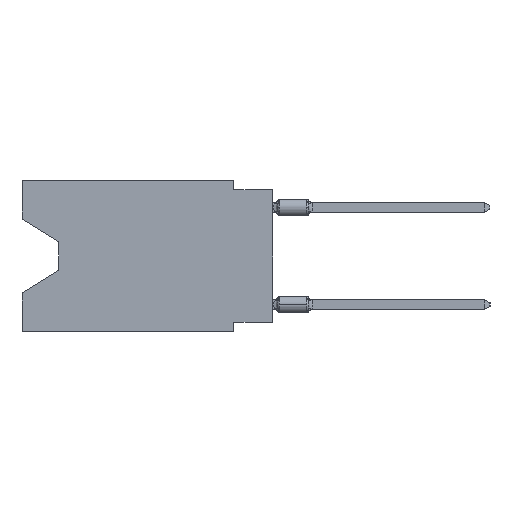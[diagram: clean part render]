
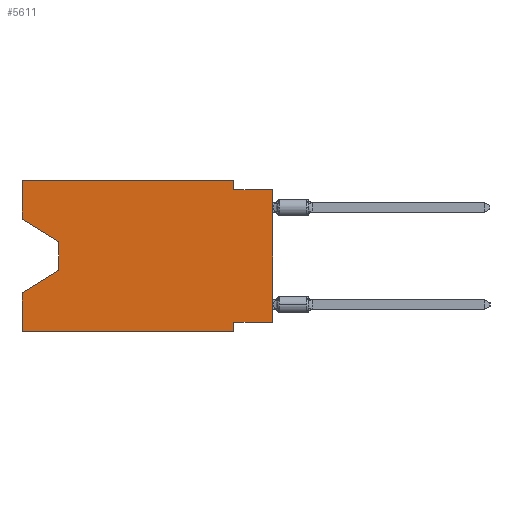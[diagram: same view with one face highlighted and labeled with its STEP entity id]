
A CAD part, left-side view. The second image highlights one B-rep face of the part: STEP entity #5611.
In plain terms, the highlighted planar face has unit normal (-1, 0, 0).
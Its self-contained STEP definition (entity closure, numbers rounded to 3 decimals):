
#142 = ORIENTED_EDGE ( 'NONE', *, *, #10924, .F. ) ;
#152 = VERTEX_POINT ( 'NONE', #18323 ) ;
#203 = VERTEX_POINT ( 'NONE', #12142 ) ;
#2177 = ORIENTED_EDGE ( 'NONE', *, *, #13288, .F. ) ;
#2533 = LINE ( 'NONE', #10088, #13872 ) ;
#2876 = DIRECTION ( 'NONE',  ( 0., 0., 1. ) ) ;
#3063 = PLANE ( 'NONE',  #28915 ) ;
#3248 = DIRECTION ( 'NONE',  ( 0., -1., 0. ) ) ;
#3420 = LINE ( 'NONE', #3580, #19638 ) ;
#3467 = CARTESIAN_POINT ( 'NONE',  ( 0., 16.383, 0. ) ) ;
#3580 = CARTESIAN_POINT ( 'NONE',  ( 0., 2.54, 0. ) ) ;
#3679 = EDGE_CURVE ( 'NONE', #25650, #23826, #5826, .T. ) ;
#4020 = VERTEX_POINT ( 'NONE', #14807 ) ;
#4327 = ORIENTED_EDGE ( 'NONE', *, *, #28011, .T. ) ;
#4393 = VECTOR ( 'NONE', #20300, 1000. ) ;
#4710 = CARTESIAN_POINT ( 'NONE',  ( 0., 2.54, -9.906 ) ) ;
#5449 = LINE ( 'NONE', #15552, #4393 ) ;
#5611 = ADVANCED_FACE ( 'NONE', ( #24685 ), #3063, .F. ) ;
#5652 = VERTEX_POINT ( 'NONE', #10784 ) ;
#5798 = VECTOR ( 'NONE', #5993, 1000. ) ;
#5826 = LINE ( 'NONE', #3467, #9163 ) ;
#5993 = DIRECTION ( 'NONE',  ( 0., 0., 1. ) ) ;
#6179 = CARTESIAN_POINT ( 'NONE',  ( 0., 16.383, 0. ) ) ;
#6827 = CARTESIAN_POINT ( 'NONE',  ( 0., 2.54, 0. ) ) ;
#7038 = ORIENTED_EDGE ( 'NONE', *, *, #7194, .F. ) ;
#7194 = EDGE_CURVE ( 'NONE', #5652, #14088, #17250, .T. ) ;
#7392 = LINE ( 'NONE', #9758, #7926 ) ;
#7404 = CARTESIAN_POINT ( 'NONE',  ( 0., 16.383, -2.546 ) ) ;
#7637 = EDGE_CURVE ( 'NONE', #27324, #152, #2533, .T. ) ;
#7926 = VECTOR ( 'NONE', #10073, 1000. ) ;
#8755 = VERTEX_POINT ( 'NONE', #20501 ) ;
#9118 = EDGE_CURVE ( 'NONE', #21921, #4020, #17063, .T. ) ;
#9163 = VECTOR ( 'NONE', #25087, 1000. ) ;
#9758 = CARTESIAN_POINT ( 'NONE',  ( 0., 0., -0.635 ) ) ;
#10073 = DIRECTION ( 'NONE',  ( 0., -1., 0. ) ) ;
#10088 = CARTESIAN_POINT ( 'NONE',  ( 0., 0., -9.271 ) ) ;
#10305 = DIRECTION ( 'NONE',  ( 0., 0., -1. ) ) ;
#10784 = CARTESIAN_POINT ( 'NONE',  ( 0., 16.383, -9.906 ) ) ;
#10878 = EDGE_CURVE ( 'NONE', #29390, #14088, #21611, .T. ) ;
#10924 = EDGE_CURVE ( 'NONE', #152, #15193, #29173, .T. ) ;
#11194 = ORIENTED_EDGE ( 'NONE', *, *, #9118, .T. ) ;
#11504 = CARTESIAN_POINT ( 'NONE',  ( 0., 13.97, -5.893 ) ) ;
#11615 = ORIENTED_EDGE ( 'NONE', *, *, #7637, .F. ) ;
#12142 = CARTESIAN_POINT ( 'NONE',  ( 0., 2.54, -0.635 ) ) ;
#12156 = DIRECTION ( 'NONE',  ( 0., 1., 0. ) ) ;
#13196 = DIRECTION ( 'NONE',  ( 0., 0., -1. ) ) ;
#13288 = EDGE_CURVE ( 'NONE', #21921, #25650, #15636, .T. ) ;
#13744 = ORIENTED_EDGE ( 'NONE', *, *, #27910, .T. ) ;
#13872 = VECTOR ( 'NONE', #12156, 1000. ) ;
#13958 = ORIENTED_EDGE ( 'NONE', *, *, #10878, .T. ) ;
#14088 = VERTEX_POINT ( 'NONE', #29305 ) ;
#14341 = DIRECTION ( 'NONE',  ( 0., 0., -1. ) ) ;
#14424 = DIRECTION ( 'NONE',  ( 0., 0., 1. ) ) ;
#14807 = CARTESIAN_POINT ( 'NONE',  ( 0., 13.97, -4.013 ) ) ;
#15193 = VERTEX_POINT ( 'NONE', #22825 ) ;
#15216 = CARTESIAN_POINT ( 'NONE',  ( 0., 16.383, 0. ) ) ;
#15418 = CARTESIAN_POINT ( 'NONE',  ( 0., 16.383, -2.546 ) ) ;
#15552 = CARTESIAN_POINT ( 'NONE',  ( 0., 13.97, -4.013 ) ) ;
#15636 = LINE ( 'NONE', #22899, #5798 ) ;
#15683 = DIRECTION ( 'NONE',  ( 1., 0., 0. ) ) ;
#16355 = VECTOR ( 'NONE', #14424, 1000. ) ;
#17034 = DIRECTION ( 'NONE',  ( 0., 0.855, -0.519 ) ) ;
#17063 = LINE ( 'NONE', #7404, #23024 ) ;
#17250 = LINE ( 'NONE', #26866, #28997 ) ;
#18003 = EDGE_CURVE ( 'NONE', #203, #8755, #7392, .T. ) ;
#18323 = CARTESIAN_POINT ( 'NONE',  ( 0., 2.54, -9.271 ) ) ;
#18401 = ORIENTED_EDGE ( 'NONE', *, *, #26496, .T. ) ;
#19637 = ORIENTED_EDGE ( 'NONE', *, *, #3679, .F. ) ;
#19638 = VECTOR ( 'NONE', #13196, 1000. ) ;
#20300 = DIRECTION ( 'NONE',  ( 0., 0., -1. ) ) ;
#20501 = CARTESIAN_POINT ( 'NONE',  ( 0., 0., -0.635 ) ) ;
#20871 = ORIENTED_EDGE ( 'NONE', *, *, #22012, .F. ) ;
#21135 = ORIENTED_EDGE ( 'NONE', *, *, #18003, .F. ) ;
#21611 = LINE ( 'NONE', #22073, #29893 ) ;
#21921 = VERTEX_POINT ( 'NONE', #15418 ) ;
#22012 = EDGE_CURVE ( 'NONE', #23826, #203, #3420, .T. ) ;
#22073 = CARTESIAN_POINT ( 'NONE',  ( 0., 13.97, -5.893 ) ) ;
#22825 = CARTESIAN_POINT ( 'NONE',  ( 0., 2.54, -9.906 ) ) ;
#22899 = CARTESIAN_POINT ( 'NONE',  ( 0., 16.383, 0. ) ) ;
#23024 = VECTOR ( 'NONE', #26673, 1000. ) ;
#23826 = VERTEX_POINT ( 'NONE', #6827 ) ;
#23898 = CARTESIAN_POINT ( 'NONE',  ( 0., 0., 0. ) ) ;
#24345 = VECTOR ( 'NONE', #14341, 1000. ) ;
#24685 = FACE_OUTER_BOUND ( 'NONE', #26416, .T. ) ;
#25087 = DIRECTION ( 'NONE',  ( 0., -1., 0. ) ) ;
#25181 = LINE ( 'NONE', #29925, #28083 ) ;
#25650 = VERTEX_POINT ( 'NONE', #6179 ) ;
#26416 = EDGE_LOOP ( 'NONE', ( #11194, #13744, #13958, #7038, #4327, #142, #11615, #18401, #21135, #20871, #19637, #2177 ) ) ;
#26496 = EDGE_CURVE ( 'NONE', #27324, #8755, #28317, .T. ) ;
#26673 = DIRECTION ( 'NONE',  ( 0., -0.855, -0.519 ) ) ;
#26866 = CARTESIAN_POINT ( 'NONE',  ( 0., 16.383, 0. ) ) ;
#27324 = VERTEX_POINT ( 'NONE', #28560 ) ;
#27910 = EDGE_CURVE ( 'NONE', #4020, #29390, #5449, .T. ) ;
#28011 = EDGE_CURVE ( 'NONE', #5652, #15193, #25181, .T. ) ;
#28083 = VECTOR ( 'NONE', #3248, 1000. ) ;
#28317 = LINE ( 'NONE', #23898, #16355 ) ;
#28560 = CARTESIAN_POINT ( 'NONE',  ( 0., 0., -9.271 ) ) ;
#28915 = AXIS2_PLACEMENT_3D ( 'NONE', #15216, #15683, #10305 ) ;
#28997 = VECTOR ( 'NONE', #2876, 1000. ) ;
#29173 = LINE ( 'NONE', #4710, #24345 ) ;
#29305 = CARTESIAN_POINT ( 'NONE',  ( 0., 16.383, -7.36 ) ) ;
#29390 = VERTEX_POINT ( 'NONE', #11504 ) ;
#29893 = VECTOR ( 'NONE', #17034, 1000. ) ;
#29925 = CARTESIAN_POINT ( 'NONE',  ( 0., 16.383, -9.906 ) ) ;
